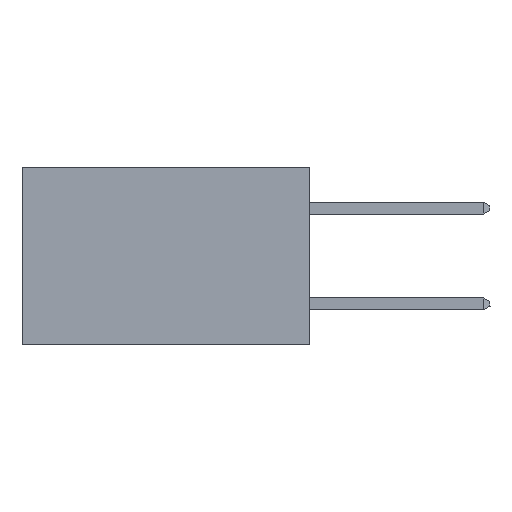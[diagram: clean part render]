
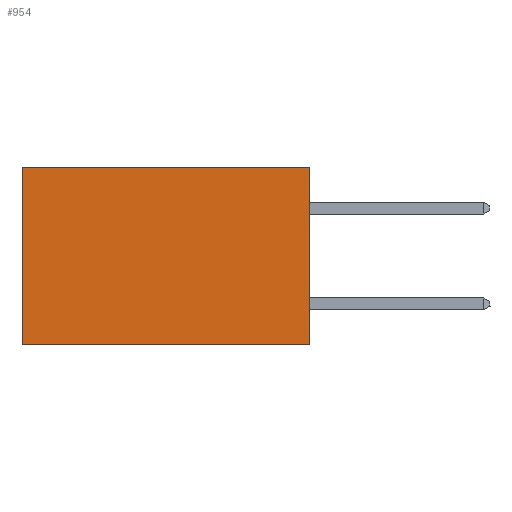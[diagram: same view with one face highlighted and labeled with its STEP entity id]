
A CAD part, left-side view. The second image highlights one B-rep face of the part: STEP entity #954.
In plain terms, the highlighted planar face has unit normal (-1, 0, 0).
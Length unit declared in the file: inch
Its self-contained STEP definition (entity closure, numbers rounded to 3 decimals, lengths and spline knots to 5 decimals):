
#292 = LINE ( 'NONE', #2443, #4670 ) ;
#941 = DIRECTION ( 'NONE',  ( 0., 1., 0. ) ) ;
#954 = ADVANCED_FACE ( 'NONE', ( #6297 ), #8126, .F. ) ;
#1356 = CARTESIAN_POINT ( 'NONE',  ( 0.2875, 0., -0.37 ) ) ;
#1433 = EDGE_CURVE ( 'NONE', #6693, #2100, #10129, .T. ) ;
#1561 = VECTOR ( 'NONE', #941, 39.37008 ) ;
#2100 = VERTEX_POINT ( 'NONE', #1356 ) ;
#2130 = AXIS2_PLACEMENT_3D ( 'NONE', #9195, #8836, #7712 ) ;
#2254 = CARTESIAN_POINT ( 'NONE',  ( 0.2875, 0.6, -0.37 ) ) ;
#2322 = LINE ( 'NONE', #8020, #10501 ) ;
#2361 = EDGE_LOOP ( 'NONE', ( #2777, #10320, #3792, #6250 ) ) ;
#2443 = CARTESIAN_POINT ( 'NONE',  ( 0.2875, 0., 0. ) ) ;
#2568 = CARTESIAN_POINT ( 'NONE',  ( 0.2875, 0., -0.37 ) ) ;
#2777 = ORIENTED_EDGE ( 'NONE', *, *, #5687, .T. ) ;
#3544 = CARTESIAN_POINT ( 'NONE',  ( 0.2875, 0., 0. ) ) ;
#3792 = ORIENTED_EDGE ( 'NONE', *, *, #1433, .F. ) ;
#4474 = EDGE_CURVE ( 'NONE', #6693, #6157, #292, .T. ) ;
#4670 = VECTOR ( 'NONE', #8195, 39.37008 ) ;
#5263 = EDGE_CURVE ( 'NONE', #2100, #6848, #10511, .T. ) ;
#5592 = DIRECTION ( 'NONE',  ( 0., 0., -1. ) ) ;
#5687 = EDGE_CURVE ( 'NONE', #6157, #6848, #2322, .T. ) ;
#6157 = VERTEX_POINT ( 'NONE', #7011 ) ;
#6250 = ORIENTED_EDGE ( 'NONE', *, *, #4474, .T. ) ;
#6297 = FACE_OUTER_BOUND ( 'NONE', #2361, .T. ) ;
#6693 = VERTEX_POINT ( 'NONE', #3544 ) ;
#6848 = VERTEX_POINT ( 'NONE', #2254 ) ;
#7011 = CARTESIAN_POINT ( 'NONE',  ( 0.2875, 0.6, 0. ) ) ;
#7712 = DIRECTION ( 'NONE',  ( 0., 0., -1. ) ) ;
#8020 = CARTESIAN_POINT ( 'NONE',  ( 0.2875, 0.6, 0. ) ) ;
#8126 = PLANE ( 'NONE',  #2130 ) ;
#8195 = DIRECTION ( 'NONE',  ( 0., 1., 0. ) ) ;
#8362 = CARTESIAN_POINT ( 'NONE',  ( 0.2875, 0., 0. ) ) ;
#8501 = DIRECTION ( 'NONE',  ( 0., 0., -1. ) ) ;
#8721 = VECTOR ( 'NONE', #8501, 39.37008 ) ;
#8836 = DIRECTION ( 'NONE',  ( 1., 0., 0. ) ) ;
#9195 = CARTESIAN_POINT ( 'NONE',  ( 0.2875, 0., 0. ) ) ;
#10129 = LINE ( 'NONE', #8362, #8721 ) ;
#10320 = ORIENTED_EDGE ( 'NONE', *, *, #5263, .F. ) ;
#10501 = VECTOR ( 'NONE', #5592, 39.37008 ) ;
#10511 = LINE ( 'NONE', #2568, #1561 ) ;
